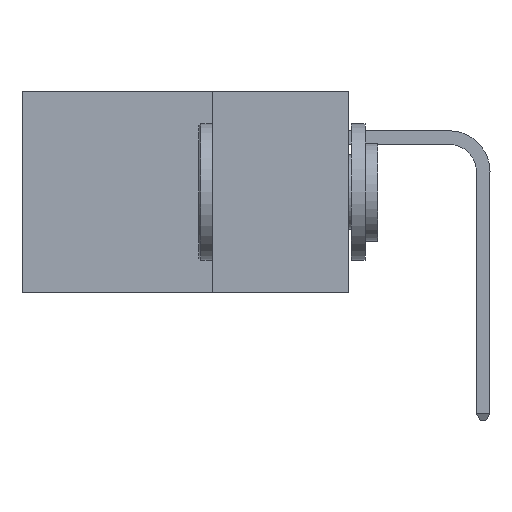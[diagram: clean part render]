
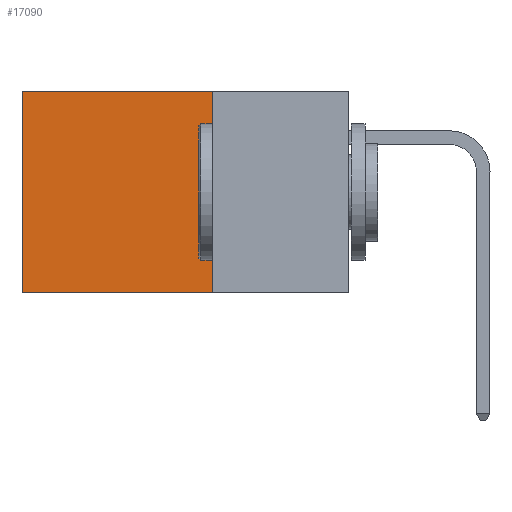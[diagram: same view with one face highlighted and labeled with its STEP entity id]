
A CAD part, left-side view. The second image highlights one B-rep face of the part: STEP entity #17090.
In plain terms, the highlighted planar face has unit normal (-1, 0, 0).
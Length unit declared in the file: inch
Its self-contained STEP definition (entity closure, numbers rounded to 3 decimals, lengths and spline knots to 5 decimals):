
#81 = CARTESIAN_POINT ( 'NONE',  ( 0.2875, 0.25, -0.37 ) ) ;
#1115 = DIRECTION ( 'NONE',  ( 0., 1., 0. ) ) ;
#4164 = ORIENTED_EDGE ( 'NONE', *, *, #25445, .F. ) ;
#4389 = DIRECTION ( 'NONE',  ( 0., 0., -1. ) ) ;
#6944 = CARTESIAN_POINT ( 'NONE',  ( 0.2875, 0.25, 0. ) ) ;
#8373 = DIRECTION ( 'NONE',  ( 0., 0., -1. ) ) ;
#8515 = LINE ( 'NONE', #26910, #14200 ) ;
#8776 = EDGE_CURVE ( 'NONE', #18692, #20177, #26746, .T. ) ;
#10351 = ORIENTED_EDGE ( 'NONE', *, *, #8776, .F. ) ;
#11398 = VECTOR ( 'NONE', #1115, 39.37008 ) ;
#11502 = CARTESIAN_POINT ( 'NONE',  ( 0.2875, 0.6, 0. ) ) ;
#12242 = AXIS2_PLACEMENT_3D ( 'NONE', #20429, #22849, #8373 ) ;
#13119 = CARTESIAN_POINT ( 'NONE',  ( 0.2875, 0.25, -0.37 ) ) ;
#13129 = PLANE ( 'NONE',  #12242 ) ;
#13719 = EDGE_LOOP ( 'NONE', ( #26234, #4164, #10351, #24260 ) ) ;
#13819 = FACE_OUTER_BOUND ( 'NONE', #13719, .T. ) ;
#14200 = VECTOR ( 'NONE', #14937, 39.37008 ) ;
#14568 = VERTEX_POINT ( 'NONE', #15646 ) ;
#14754 = EDGE_CURVE ( 'NONE', #14568, #20743, #20036, .T. ) ;
#14937 = DIRECTION ( 'NONE',  ( 0., 1., 0. ) ) ;
#15646 = CARTESIAN_POINT ( 'NONE',  ( 0.2875, 0.6, 0. ) ) ;
#16307 = CARTESIAN_POINT ( 'NONE',  ( 0.2875, 0.25, 0. ) ) ;
#17090 = ADVANCED_FACE ( 'NONE', ( #13819 ), #13129, .F. ) ;
#18692 = VERTEX_POINT ( 'NONE', #6944 ) ;
#19287 = VECTOR ( 'NONE', #23544, 39.37008 ) ;
#19356 = LINE ( 'NONE', #13119, #11398 ) ;
#20036 = LINE ( 'NONE', #11502, #19287 ) ;
#20177 = VERTEX_POINT ( 'NONE', #81 ) ;
#20429 = CARTESIAN_POINT ( 'NONE',  ( 0.2875, 0.25, 0. ) ) ;
#20743 = VERTEX_POINT ( 'NONE', #26058 ) ;
#22849 = DIRECTION ( 'NONE',  ( 1., 0., 0. ) ) ;
#23399 = EDGE_CURVE ( 'NONE', #18692, #14568, #8515, .T. ) ;
#23544 = DIRECTION ( 'NONE',  ( 0., 0., -1. ) ) ;
#24260 = ORIENTED_EDGE ( 'NONE', *, *, #23399, .T. ) ;
#25445 = EDGE_CURVE ( 'NONE', #20177, #20743, #19356, .T. ) ;
#25998 = VECTOR ( 'NONE', #4389, 39.37008 ) ;
#26058 = CARTESIAN_POINT ( 'NONE',  ( 0.2875, 0.6, -0.37 ) ) ;
#26234 = ORIENTED_EDGE ( 'NONE', *, *, #14754, .T. ) ;
#26746 = LINE ( 'NONE', #16307, #25998 ) ;
#26910 = CARTESIAN_POINT ( 'NONE',  ( 0.2875, 0.25, 0. ) ) ;
